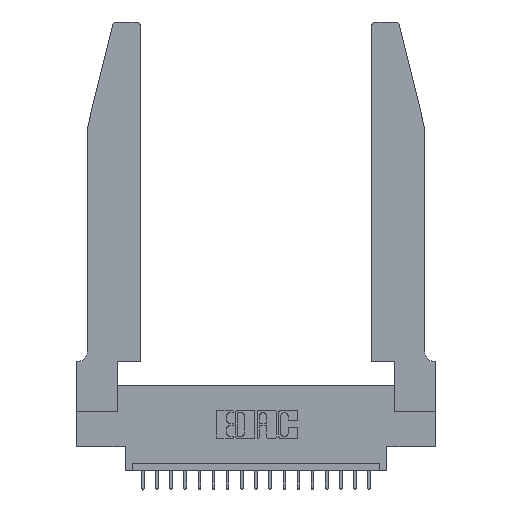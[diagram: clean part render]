
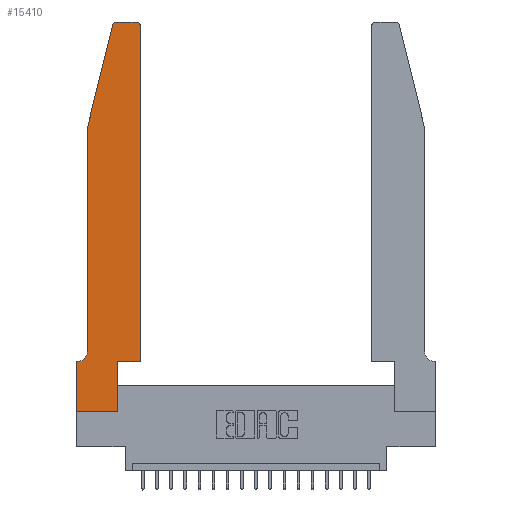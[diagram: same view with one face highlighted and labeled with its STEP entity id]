
A CAD part, top view. The second image highlights one B-rep face of the part: STEP entity #15410.
In plain terms, the highlighted planar face has unit normal (0, 0, 1).
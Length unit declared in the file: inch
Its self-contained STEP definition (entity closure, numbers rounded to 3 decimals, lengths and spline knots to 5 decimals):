
#21 = CARTESIAN_POINT ( 'NONE',  ( 0.2605, 2.75, 0.37 ) ) ;
#369 = VECTOR ( 'NONE', #3915, 39.37008 ) ;
#432 = CARTESIAN_POINT ( 'NONE',  ( 0., 0., 0.37 ) ) ;
#564 = VERTEX_POINT ( 'NONE', #17961 ) ;
#1584 = ORIENTED_EDGE ( 'NONE', *, *, #13352, .T. ) ;
#1592 = VERTEX_POINT ( 'NONE', #15282 ) ;
#1603 = VERTEX_POINT ( 'NONE', #13783 ) ;
#1638 = LINE ( 'NONE', #21, #7661 ) ;
#1925 = DIRECTION ( 'NONE',  ( 1., 0., 0. ) ) ;
#2210 = VECTOR ( 'NONE', #8430, 39.37008 ) ;
#2550 = DIRECTION ( 'NONE',  ( 0., 0., 1. ) ) ;
#2842 = CARTESIAN_POINT ( 'NONE',  ( 0., 0.35, 0.37 ) ) ;
#2881 = EDGE_CURVE ( 'NONE', #1603, #15872, #8722, .T. ) ;
#3443 = LINE ( 'NONE', #4823, #2210 ) ;
#3696 = LINE ( 'NONE', #13712, #369 ) ;
#3757 = CARTESIAN_POINT ( 'NONE',  ( 0.4505, 0.35, 0.37 ) ) ;
#3785 = ORIENTED_EDGE ( 'NONE', *, *, #9917, .T. ) ;
#3915 = DIRECTION ( 'NONE',  ( -0.239, -0.971, 0. ) ) ;
#4142 = VERTEX_POINT ( 'NONE', #20072 ) ;
#4289 = DIRECTION ( 'NONE',  ( 1., 0., 0. ) ) ;
#4427 = LINE ( 'NONE', #18022, #14869 ) ;
#4434 = PLANE ( 'NONE',  #17348 ) ;
#4579 = VECTOR ( 'NONE', #4289, 39.37008 ) ;
#4823 = CARTESIAN_POINT ( 'NONE',  ( 0.2865, 0.35, 0.37 ) ) ;
#5202 = VERTEX_POINT ( 'NONE', #20103 ) ;
#6224 = DIRECTION ( 'NONE',  ( 0., 0., 1. ) ) ;
#6290 = CIRCLE ( 'NONE', #18212, 0.07 ) ;
#6365 = CARTESIAN_POINT ( 'NONE',  ( 0., 0., 0.37 ) ) ;
#6421 = VECTOR ( 'NONE', #1925, 39.37008 ) ;
#6439 = CIRCLE ( 'NONE', #10191, 0.03 ) ;
#6540 = DIRECTION ( 'NONE',  ( -1., 0., 0. ) ) ;
#6855 = VECTOR ( 'NONE', #8677, 39.37008 ) ;
#7661 = VECTOR ( 'NONE', #6540, 39.37008 ) ;
#7684 = CARTESIAN_POINT ( 'NONE',  ( 0.4505, 0.35, 0.37 ) ) ;
#8430 = DIRECTION ( 'NONE',  ( 0., 1., 0. ) ) ;
#8468 = LINE ( 'NONE', #16712, #6855 ) ;
#8581 = VERTEX_POINT ( 'NONE', #6365 ) ;
#8677 = DIRECTION ( 'NONE',  ( -1., 0., 0. ) ) ;
#8722 = LINE ( 'NONE', #18649, #11664 ) ;
#9043 = DIRECTION ( 'NONE',  ( 1., 0., 0. ) ) ;
#9112 = DIRECTION ( 'NONE',  ( 1., 0., 0. ) ) ;
#9156 = VERTEX_POINT ( 'NONE', #15080 ) ;
#9251 = ORIENTED_EDGE ( 'NONE', *, *, #19740, .T. ) ;
#9332 = FACE_OUTER_BOUND ( 'NONE', #10872, .T. ) ;
#9402 = EDGE_CURVE ( 'NONE', #14632, #4142, #4427, .T. ) ;
#9428 = AXIS2_PLACEMENT_3D ( 'NONE', #18975, #2550, #9043 ) ;
#9635 = EDGE_CURVE ( 'NONE', #564, #18652, #16266, .T. ) ;
#9906 = VERTEX_POINT ( 'NONE', #18511 ) ;
#9917 = EDGE_CURVE ( 'NONE', #18652, #1603, #3696, .T. ) ;
#10030 = LINE ( 'NONE', #17930, #6421 ) ;
#10100 = ORIENTED_EDGE ( 'NONE', *, *, #18005, .T. ) ;
#10165 = LINE ( 'NONE', #432, #18030 ) ;
#10191 = AXIS2_PLACEMENT_3D ( 'NONE', #20759, #19032, #9112 ) ;
#10518 = ORIENTED_EDGE ( 'NONE', *, *, #18255, .T. ) ;
#10872 = EDGE_LOOP ( 'NONE', ( #9251, #18224, #3785, #15840, #1584, #10100, #17679, #18468, #11486, #11390, #20899, #10518 ) ) ;
#11145 = DIRECTION ( 'NONE',  ( -1., 0., 0. ) ) ;
#11390 = ORIENTED_EDGE ( 'NONE', *, *, #12389, .T. ) ;
#11486 = ORIENTED_EDGE ( 'NONE', *, *, #13392, .T. ) ;
#11664 = VECTOR ( 'NONE', #20485, 39.37008 ) ;
#12389 = EDGE_CURVE ( 'NONE', #5202, #14632, #13871, .T. ) ;
#12715 = CARTESIAN_POINT ( 'NONE',  ( 0.0755, 0.42, 0.37 ) ) ;
#12835 = CARTESIAN_POINT ( 'NONE',  ( 0.0055, 0.42, 0.37 ) ) ;
#13352 = EDGE_CURVE ( 'NONE', #15872, #1592, #6290, .T. ) ;
#13392 = EDGE_CURVE ( 'NONE', #19112, #5202, #3443, .T. ) ;
#13712 = CARTESIAN_POINT ( 'NONE',  ( 0.0755, 2., 0.37 ) ) ;
#13783 = CARTESIAN_POINT ( 'NONE',  ( 0.0755, 2., 0.37 ) ) ;
#13871 = LINE ( 'NONE', #7684, #4579 ) ;
#14440 = DIRECTION ( 'NONE',  ( 0., 0., -1. ) ) ;
#14632 = VERTEX_POINT ( 'NONE', #3757 ) ;
#14869 = VECTOR ( 'NONE', #19229, 39.37008 ) ;
#14917 = EDGE_CURVE ( 'NONE', #8581, #19112, #10030, .T. ) ;
#14956 = DIRECTION ( 'NONE',  ( 0., -1., 0. ) ) ;
#15080 = CARTESIAN_POINT ( 'NONE',  ( 0.4205, 2.75, 0.37 ) ) ;
#15282 = CARTESIAN_POINT ( 'NONE',  ( 0.0055, 0.35, 0.37 ) ) ;
#15410 = ADVANCED_FACE ( 'NONE', ( #9332 ), #4434, .T. ) ;
#15636 = EDGE_CURVE ( 'NONE', #9906, #8581, #10165, .T. ) ;
#15840 = ORIENTED_EDGE ( 'NONE', *, *, #2881, .T. ) ;
#15872 = VERTEX_POINT ( 'NONE', #12715 ) ;
#16266 = CIRCLE ( 'NONE', #9428, 0.03 ) ;
#16712 = CARTESIAN_POINT ( 'NONE',  ( 0.0755, 0.35, 0.37 ) ) ;
#17348 = AXIS2_PLACEMENT_3D ( 'NONE', #2842, #6224, #19144 ) ;
#17679 = ORIENTED_EDGE ( 'NONE', *, *, #15636, .T. ) ;
#17930 = CARTESIAN_POINT ( 'NONE',  ( 0., 0., 0.37 ) ) ;
#17961 = CARTESIAN_POINT ( 'NONE',  ( 0.284, 2.75, 0.37 ) ) ;
#18005 = EDGE_CURVE ( 'NONE', #1592, #9906, #8468, .T. ) ;
#18022 = CARTESIAN_POINT ( 'NONE',  ( 0.4505, 0.35, 0.37 ) ) ;
#18030 = VECTOR ( 'NONE', #14956, 39.37008 ) ;
#18212 = AXIS2_PLACEMENT_3D ( 'NONE', #12835, #14440, #11145 ) ;
#18224 = ORIENTED_EDGE ( 'NONE', *, *, #9635, .T. ) ;
#18255 = EDGE_CURVE ( 'NONE', #4142, #9156, #6439, .T. ) ;
#18468 = ORIENTED_EDGE ( 'NONE', *, *, #14917, .T. ) ;
#18511 = CARTESIAN_POINT ( 'NONE',  ( 0., 0.35, 0.37 ) ) ;
#18649 = CARTESIAN_POINT ( 'NONE',  ( 0.0755, 2., 0.37 ) ) ;
#18652 = VERTEX_POINT ( 'NONE', #19118 ) ;
#18657 = CARTESIAN_POINT ( 'NONE',  ( 0.2865, 0., 0.37 ) ) ;
#18975 = CARTESIAN_POINT ( 'NONE',  ( 0.284, 2.72, 0.37 ) ) ;
#19032 = DIRECTION ( 'NONE',  ( 0., 0., 1. ) ) ;
#19112 = VERTEX_POINT ( 'NONE', #18657 ) ;
#19118 = CARTESIAN_POINT ( 'NONE',  ( 0.25487, 2.72718, 0.37 ) ) ;
#19144 = DIRECTION ( 'NONE',  ( 1., 0., 0. ) ) ;
#19229 = DIRECTION ( 'NONE',  ( 0., 1., 0. ) ) ;
#19740 = EDGE_CURVE ( 'NONE', #9156, #564, #1638, .T. ) ;
#20072 = CARTESIAN_POINT ( 'NONE',  ( 0.4505, 2.72, 0.37 ) ) ;
#20103 = CARTESIAN_POINT ( 'NONE',  ( 0.2865, 0.35, 0.37 ) ) ;
#20485 = DIRECTION ( 'NONE',  ( 0., -1., 0. ) ) ;
#20759 = CARTESIAN_POINT ( 'NONE',  ( 0.4205, 2.72, 0.37 ) ) ;
#20899 = ORIENTED_EDGE ( 'NONE', *, *, #9402, .T. ) ;
